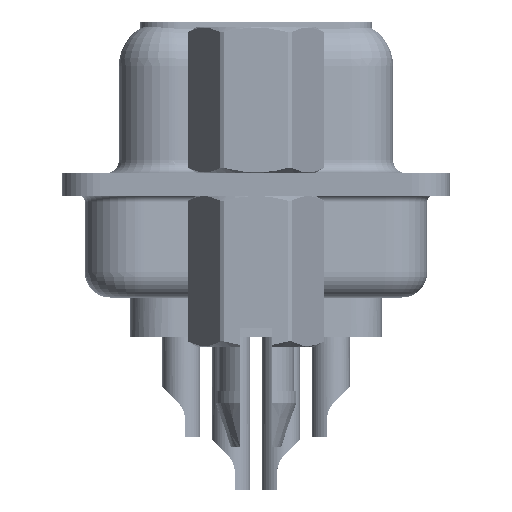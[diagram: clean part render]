
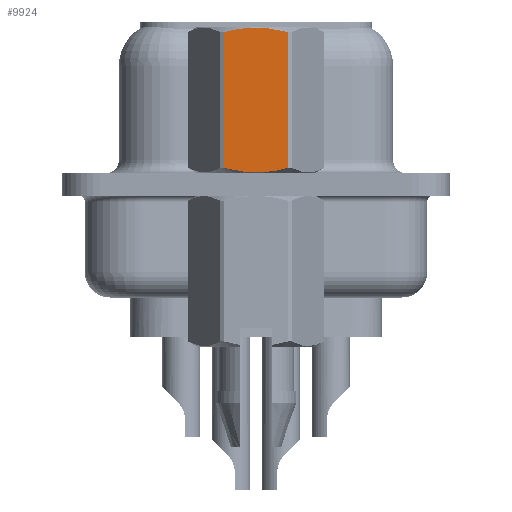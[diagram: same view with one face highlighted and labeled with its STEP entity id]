
A CAD part, left-side view. The second image highlights one B-rep face of the part: STEP entity #9924.
In plain terms, the highlighted planar face has unit normal (-1, 0, 0).
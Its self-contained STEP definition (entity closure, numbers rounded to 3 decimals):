
#538 = ORIENTED_EDGE ( 'NONE', *, *, #45760, .T. ) ;
#4233 = CARTESIAN_POINT ( 'NONE',  ( -2.381, 1.273, 0.652 ) ) ;
#4798 = CARTESIAN_POINT ( 'NONE',  ( -2.381, -0.432, 0.485 ) ) ;
#9189 = B_SPLINE_CURVE_WITH_KNOTS ( 'NONE', 3,
 ( #4233, #45435, #36508, #54652, #46027, #18701, #4798, #23440, #32342, #40706 ),
 .UNSPECIFIED., .F., .F.,
 ( 4, 2, 2, 2, 4 ),
 ( 0.003, 0.003, 0.004, 0.004, 0.005 ),
 .UNSPECIFIED. ) ;
#9924 = ADVANCED_FACE ( 'NONE', ( #15308 ), #29231, .T. ) ;
#15308 = FACE_OUTER_BOUND ( 'NONE', #33495, .T. ) ;
#15491 = ORIENTED_EDGE ( 'NONE', *, *, #23167, .T. ) ;
#16545 = VERTEX_POINT ( 'NONE', #22024 ) ;
#18406 = VERTEX_POINT ( 'NONE', #18957 ) ;
#18701 = CARTESIAN_POINT ( 'NONE',  ( -2.381, -0.215, 0.468 ) ) ;
#18830 = DIRECTION ( 'NONE',  ( 0., 0., -1. ) ) ;
#18932 = CARTESIAN_POINT ( 'NONE',  ( -2.381, -1.273, 6.048 ) ) ;
#18957 = CARTESIAN_POINT ( 'NONE',  ( -2.381, -1.273, 0.652 ) ) ;
#22024 = CARTESIAN_POINT ( 'NONE',  ( -2.381, 1.273, 6.048 ) ) ;
#22475 = DIRECTION ( 'NONE',  ( 0., 0., 1. ) ) ;
#22531 = DIRECTION ( 'NONE',  ( -1., 0., 0. ) ) ;
#23167 = EDGE_CURVE ( 'NONE', #16545, #30307, #37789, .T. ) ;
#23440 = CARTESIAN_POINT ( 'NONE',  ( -2.381, -0.858, 0.55 ) ) ;
#23802 = EDGE_CURVE ( 'NONE', #45215, #16545, #48065, .T. ) ;
#24483 = VECTOR ( 'NONE', #22475, 1000. ) ;
#26931 = AXIS2_PLACEMENT_3D ( 'NONE', #56286, #22531, #55691 ) ;
#29231 = PLANE ( 'NONE',  #26931 ) ;
#29668 = VECTOR ( 'NONE', #18830, 1000. ) ;
#30307 = VERTEX_POINT ( 'NONE', #36339 ) ;
#30592 = CARTESIAN_POINT ( 'NONE',  ( -2.381, 1.273, 6.048 ) ) ;
#31185 = CARTESIAN_POINT ( 'NONE',  ( -2.381, -0.858, 6.15 ) ) ;
#31469 = CARTESIAN_POINT ( 'NONE',  ( -2.381, 0.428, 6.215 ) ) ;
#31759 = CARTESIAN_POINT ( 'NONE',  ( -2.381, 0.215, 6.232 ) ) ;
#32342 = CARTESIAN_POINT ( 'NONE',  ( -2.381, -1.066, 0.596 ) ) ;
#33495 = EDGE_LOOP ( 'NONE', ( #48707, #538, #53944, #15491 ) ) ;
#33648 = CARTESIAN_POINT ( 'NONE',  ( -2.381, 1.273, 3.792 ) ) ;
#36211 = CARTESIAN_POINT ( 'NONE',  ( -2.381, -1.273, 6.048 ) ) ;
#36339 = CARTESIAN_POINT ( 'NONE',  ( -2.381, 1.273, 0.652 ) ) ;
#36508 = CARTESIAN_POINT ( 'NONE',  ( -2.381, 0.853, 0.549 ) ) ;
#37789 = LINE ( 'NONE', #33648, #29668 ) ;
#39832 = CARTESIAN_POINT ( 'NONE',  ( -2.381, -1.066, 6.104 ) ) ;
#40419 = CARTESIAN_POINT ( 'NONE',  ( -2.381, 0.853, 6.151 ) ) ;
#40706 = CARTESIAN_POINT ( 'NONE',  ( -2.381, -1.273, 0.652 ) ) ;
#40889 = LINE ( 'NONE', #45623, #24483 ) ;
#45215 = VERTEX_POINT ( 'NONE', #18932 ) ;
#45435 = CARTESIAN_POINT ( 'NONE',  ( -2.381, 1.065, 0.596 ) ) ;
#45623 = CARTESIAN_POINT ( 'NONE',  ( -2.381, -1.273, 3.792 ) ) ;
#45760 = EDGE_CURVE ( 'NONE', #18406, #45215, #40889, .T. ) ;
#46027 = CARTESIAN_POINT ( 'NONE',  ( -2.381, 0.215, 0.468 ) ) ;
#48065 = B_SPLINE_CURVE_WITH_KNOTS ( 'NONE', 3,
 ( #36211, #39832, #31185, #49917, #54068, #31759, #31469, #40419, #49337, #30592 ),
 .UNSPECIFIED., .F., .F.,
 ( 4, 2, 2, 2, 4 ),
 ( 0.001, 0.002, 0.002, 0.003, 0.004 ),
 .UNSPECIFIED. ) ;
#48707 = ORIENTED_EDGE ( 'NONE', *, *, #49567, .T. ) ;
#49337 = CARTESIAN_POINT ( 'NONE',  ( -2.381, 1.065, 6.104 ) ) ;
#49567 = EDGE_CURVE ( 'NONE', #30307, #18406, #9189, .T. ) ;
#49917 = CARTESIAN_POINT ( 'NONE',  ( -2.381, -0.432, 6.215 ) ) ;
#53944 = ORIENTED_EDGE ( 'NONE', *, *, #23802, .T. ) ;
#54068 = CARTESIAN_POINT ( 'NONE',  ( -2.381, -0.215, 6.232 ) ) ;
#54652 = CARTESIAN_POINT ( 'NONE',  ( -2.381, 0.428, 0.485 ) ) ;
#55691 = DIRECTION ( 'NONE',  ( 0., -1., 0. ) ) ;
#56286 = CARTESIAN_POINT ( 'NONE',  ( -2.381, 1.375, -3.75 ) ) ;
